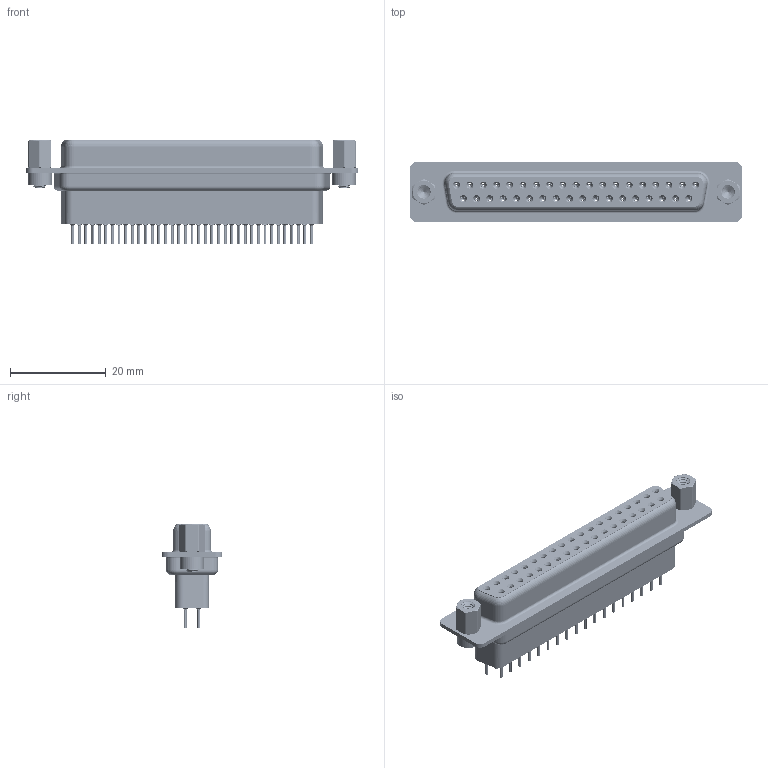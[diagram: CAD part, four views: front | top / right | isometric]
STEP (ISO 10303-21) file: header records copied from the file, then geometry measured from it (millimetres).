
FILE_DESCRIPTION (( 'STEP AP203' ), '1' );
FILE_NAME ('628-037-621-073.STEP', '2020-07-14T20:39:42', ( '' ), ( '' ), 'SwSTEP 2.0', 'SolidWorks 2020', '' );
FILE_SCHEMA (( 'CONFIG_CONTROL_DESIGN' ));
Length unit declared in the file: millimetre
Products named in the file (8): 628-037-621-073; 628 Shell Front_37 Contacts; 628 Contact Row 2_21H; 628 Shell Rear_37 Contacts; 628 Housing_37 HP; 628 Contact Row 1_21H; 628 4-40 Hex Standoff; 628 4-40 Threaded Rivet
Assembly tree (44 placements, depth 2):
  628-037-621-073
    628 Housing_37 HP
    628 Shell Front_37 Contacts
    628 Shell Rear_37 Contacts
    628 Contact Row 1_21H  x19
    628 Contact Row 2_21H  x18
    628 4-40 Threaded Rivet  x2
    628 4-40 Hex Standoff  x2
Bounding box: 69.3 x 12.6 x 21.9 mm (x, y, z)
Volume: 7239.8 mm3; surface area: 16539.5 mm2
Topology: 44 solids, 44 shells, 4952 faces, 12715 edges, 7936 vertices
Faces by surface type: cylinder 1428, plane 1236, torus 945, bspline 758, cone 585
Entity records: 37319 total; most frequent: CARTESIAN_POINT 11837, DIRECTION 5215, ORIENTED_EDGE 4762, EDGE_CURVE 2381, AXIS2_PLACEMENT_3D 2188, VERTEX_POINT 1509, EDGE_LOOP 1218, CIRCLE 1182
